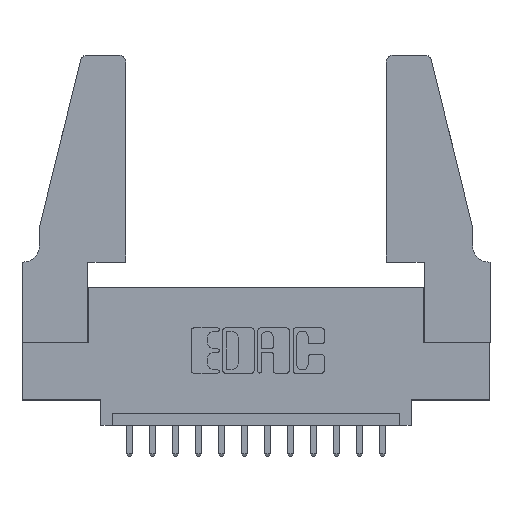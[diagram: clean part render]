
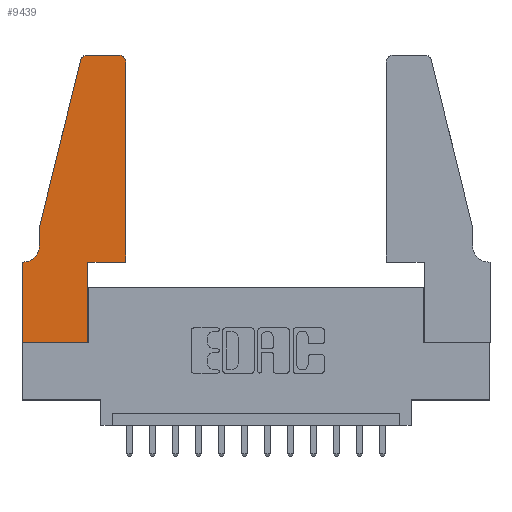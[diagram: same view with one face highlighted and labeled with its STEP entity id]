
A CAD part, top view. The second image highlights one B-rep face of the part: STEP entity #9439.
In plain terms, the highlighted planar face has unit normal (0, 0, 1).
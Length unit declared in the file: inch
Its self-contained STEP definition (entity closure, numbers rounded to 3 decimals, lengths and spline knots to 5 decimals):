
#138 = VERTEX_POINT ( 'NONE', #14938 ) ;
#581 = LINE ( 'NONE', #10898, #13970 ) ;
#585 = CARTESIAN_POINT ( 'NONE',  ( 0.0755, 0.35, 0.37 ) ) ;
#1023 = VECTOR ( 'NONE', #8287, 39.37008 ) ;
#1036 = EDGE_CURVE ( 'NONE', #4154, #2467, #13597, .T. ) ;
#1243 = DIRECTION ( 'NONE',  ( 0., 0., 1. ) ) ;
#1401 = LINE ( 'NONE', #7226, #2157 ) ;
#1670 = CIRCLE ( 'NONE', #11256, 0.03 ) ;
#1848 = ORIENTED_EDGE ( 'NONE', *, *, #5951, .T. ) ;
#2157 = VECTOR ( 'NONE', #3784, 39.37008 ) ;
#2258 = ORIENTED_EDGE ( 'NONE', *, *, #3713, .T. ) ;
#2260 = ORIENTED_EDGE ( 'NONE', *, *, #14587, .T. ) ;
#2467 = VERTEX_POINT ( 'NONE', #13658 ) ;
#2499 = CARTESIAN_POINT ( 'NONE',  ( 0., 0., 0.37 ) ) ;
#2723 = EDGE_LOOP ( 'NONE', ( #13137, #8554, #11126, #2258, #10202, #14765, #14499, #14787, #2842, #1848, #5280, #2260 ) ) ;
#2842 = ORIENTED_EDGE ( 'NONE', *, *, #5188, .T. ) ;
#3031 = AXIS2_PLACEMENT_3D ( 'NONE', #11026, #8574, #6339 ) ;
#3211 = VECTOR ( 'NONE', #7802, 39.37008 ) ;
#3224 = VERTEX_POINT ( 'NONE', #6809 ) ;
#3713 = EDGE_CURVE ( 'NONE', #2467, #9958, #14432, .T. ) ;
#3784 = DIRECTION ( 'NONE',  ( 0., 1., 0. ) ) ;
#3800 = EDGE_CURVE ( 'NONE', #9447, #8363, #9997, .T. ) ;
#3823 = VERTEX_POINT ( 'NONE', #6673 ) ;
#4154 = VERTEX_POINT ( 'NONE', #13126 ) ;
#4193 = CARTESIAN_POINT ( 'NONE',  ( 0.0755, 0.42, 0.37 ) ) ;
#4431 = CARTESIAN_POINT ( 'NONE',  ( 0.4505, 0.35, 0.37 ) ) ;
#4472 = VECTOR ( 'NONE', #11674, 39.37008 ) ;
#4875 = LINE ( 'NONE', #9957, #9152 ) ;
#5188 = EDGE_CURVE ( 'NONE', #9646, #14285, #1401, .T. ) ;
#5280 = ORIENTED_EDGE ( 'NONE', *, *, #11993, .T. ) ;
#5440 = DIRECTION ( 'NONE',  ( 1., 0., 0. ) ) ;
#5493 = CIRCLE ( 'NONE', #8196, 0.03 ) ;
#5560 = DIRECTION ( 'NONE',  ( 1., 0., 0. ) ) ;
#5576 = EDGE_CURVE ( 'NONE', #9810, #9646, #15314, .T. ) ;
#5801 = EDGE_CURVE ( 'NONE', #3224, #14229, #4875, .T. ) ;
#5858 = CARTESIAN_POINT ( 'NONE',  ( 0.2865, 0.35, 0.37 ) ) ;
#5951 = EDGE_CURVE ( 'NONE', #14285, #138, #13014, .T. ) ;
#6161 = DIRECTION ( 'NONE',  ( 0., -1., 0. ) ) ;
#6339 = DIRECTION ( 'NONE',  ( -1., 0., 0. ) ) ;
#6673 = CARTESIAN_POINT ( 'NONE',  ( 0.4505, 1.22, 0.37 ) ) ;
#6809 = CARTESIAN_POINT ( 'NONE',  ( 0.4205, 1.25, 0.37 ) ) ;
#6826 = VECTOR ( 'NONE', #8926, 39.37008 ) ;
#6947 = EDGE_CURVE ( 'NONE', #14229, #4154, #1670, .T. ) ;
#7226 = CARTESIAN_POINT ( 'NONE',  ( 0.2865, 0.35, 0.37 ) ) ;
#7602 = DIRECTION ( 'NONE',  ( -1., 0., 0. ) ) ;
#7802 = DIRECTION ( 'NONE',  ( 1., 0., 0. ) ) ;
#8113 = CARTESIAN_POINT ( 'NONE',  ( 0., 0.35, 0.37 ) ) ;
#8196 = AXIS2_PLACEMENT_3D ( 'NONE', #12027, #10340, #5440 ) ;
#8287 = DIRECTION ( 'NONE',  ( 1., 0., 0. ) ) ;
#8353 = CARTESIAN_POINT ( 'NONE',  ( 0.284, 1.22, 0.37 ) ) ;
#8363 = VERTEX_POINT ( 'NONE', #15261 ) ;
#8554 = ORIENTED_EDGE ( 'NONE', *, *, #6947, .T. ) ;
#8574 = DIRECTION ( 'NONE',  ( 0., 0., -1. ) ) ;
#8857 = FACE_OUTER_BOUND ( 'NONE', #2723, .T. ) ;
#8926 = DIRECTION ( 'NONE',  ( -1., 0., 0. ) ) ;
#8989 = AXIS2_PLACEMENT_3D ( 'NONE', #8113, #10279, #5560 ) ;
#8992 = CARTESIAN_POINT ( 'NONE',  ( 0.284, 1.25, 0.37 ) ) ;
#9152 = VECTOR ( 'NONE', #7602, 39.37008 ) ;
#9439 = ADVANCED_FACE ( 'NONE', ( #8857 ), #15223, .T. ) ;
#9447 = VERTEX_POINT ( 'NONE', #14849 ) ;
#9646 = VERTEX_POINT ( 'NONE', #12983 ) ;
#9810 = VERTEX_POINT ( 'NONE', #2499 ) ;
#9957 = CARTESIAN_POINT ( 'NONE',  ( 0.2605, 1.25, 0.37 ) ) ;
#9958 = VERTEX_POINT ( 'NONE', #4193 ) ;
#9997 = LINE ( 'NONE', #585, #6826 ) ;
#10187 = EDGE_CURVE ( 'NONE', #9958, #9447, #11031, .T. ) ;
#10202 = ORIENTED_EDGE ( 'NONE', *, *, #10187, .T. ) ;
#10279 = DIRECTION ( 'NONE',  ( 0., 0., 1. ) ) ;
#10340 = DIRECTION ( 'NONE',  ( 0., 0., 1. ) ) ;
#10701 = DIRECTION ( 'NONE',  ( 1., 0., 0. ) ) ;
#10757 = CARTESIAN_POINT ( 'NONE',  ( 0.0755, 0.5, 0.37 ) ) ;
#10898 = CARTESIAN_POINT ( 'NONE',  ( 0.4505, 0.35, 0.37 ) ) ;
#11026 = CARTESIAN_POINT ( 'NONE',  ( 0.0055, 0.42, 0.37 ) ) ;
#11031 = CIRCLE ( 'NONE', #3031, 0.07 ) ;
#11126 = ORIENTED_EDGE ( 'NONE', *, *, #1036, .T. ) ;
#11256 = AXIS2_PLACEMENT_3D ( 'NONE', #8353, #1243, #10701 ) ;
#11674 = DIRECTION ( 'NONE',  ( 0., -1., 0. ) ) ;
#11993 = EDGE_CURVE ( 'NONE', #138, #3823, #581, .T. ) ;
#12027 = CARTESIAN_POINT ( 'NONE',  ( 0.4205, 1.22, 0.37 ) ) ;
#12420 = LINE ( 'NONE', #14518, #4472 ) ;
#12551 = EDGE_CURVE ( 'NONE', #8363, #9810, #12420, .T. ) ;
#12983 = CARTESIAN_POINT ( 'NONE',  ( 0.2865, 0., 0.37 ) ) ;
#13014 = LINE ( 'NONE', #4431, #3211 ) ;
#13126 = CARTESIAN_POINT ( 'NONE',  ( 0.25487, 1.22718, 0.37 ) ) ;
#13137 = ORIENTED_EDGE ( 'NONE', *, *, #5801, .T. ) ;
#13175 = DIRECTION ( 'NONE',  ( -0.239, -0.971, 0. ) ) ;
#13256 = DIRECTION ( 'NONE',  ( 0., 1., 0. ) ) ;
#13310 = VECTOR ( 'NONE', #6161, 39.37008 ) ;
#13597 = LINE ( 'NONE', #10757, #14510 ) ;
#13658 = CARTESIAN_POINT ( 'NONE',  ( 0.0755, 0.5, 0.37 ) ) ;
#13970 = VECTOR ( 'NONE', #13256, 39.37008 ) ;
#14229 = VERTEX_POINT ( 'NONE', #8992 ) ;
#14285 = VERTEX_POINT ( 'NONE', #5858 ) ;
#14432 = LINE ( 'NONE', #14604, #13310 ) ;
#14499 = ORIENTED_EDGE ( 'NONE', *, *, #12551, .T. ) ;
#14510 = VECTOR ( 'NONE', #13175, 39.37008 ) ;
#14518 = CARTESIAN_POINT ( 'NONE',  ( 0., 0., 0.37 ) ) ;
#14587 = EDGE_CURVE ( 'NONE', #3823, #3224, #5493, .T. ) ;
#14604 = CARTESIAN_POINT ( 'NONE',  ( 0.0755, 0.5, 0.37 ) ) ;
#14765 = ORIENTED_EDGE ( 'NONE', *, *, #3800, .T. ) ;
#14787 = ORIENTED_EDGE ( 'NONE', *, *, #5576, .T. ) ;
#14849 = CARTESIAN_POINT ( 'NONE',  ( 0.0055, 0.35, 0.37 ) ) ;
#14938 = CARTESIAN_POINT ( 'NONE',  ( 0.4505, 0.35, 0.37 ) ) ;
#15223 = PLANE ( 'NONE',  #8989 ) ;
#15261 = CARTESIAN_POINT ( 'NONE',  ( 0., 0.35, 0.37 ) ) ;
#15314 = LINE ( 'NONE', #15388, #1023 ) ;
#15388 = CARTESIAN_POINT ( 'NONE',  ( 0., 0., 0.37 ) ) ;
